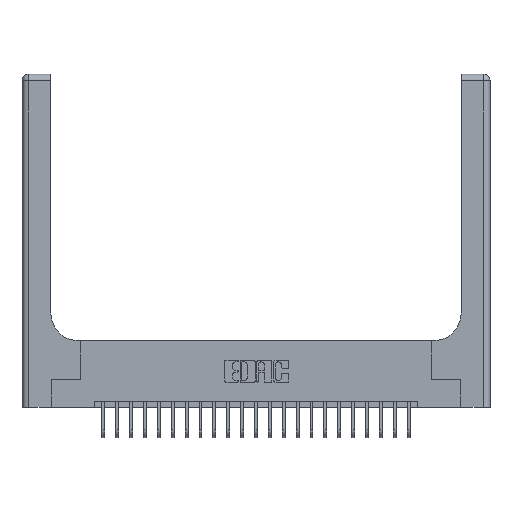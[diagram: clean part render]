
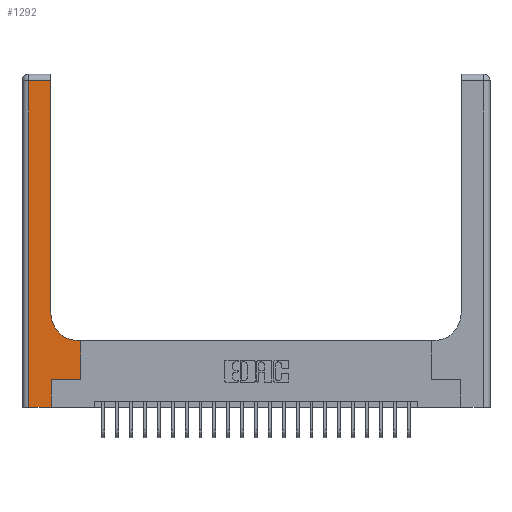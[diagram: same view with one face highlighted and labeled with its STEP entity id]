
A CAD part, top view. The second image highlights one B-rep face of the part: STEP entity #1292.
In plain terms, the highlighted planar face has unit normal (0, 0, 1).
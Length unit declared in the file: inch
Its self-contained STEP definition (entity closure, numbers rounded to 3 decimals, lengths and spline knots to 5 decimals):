
#1076 = DIRECTION ( 'NONE',  ( 0., 1., 0. ) ) ;
#1092 = EDGE_CURVE ( 'NONE', #19050, #2281, #2608, .T. ) ;
#1292 = ADVANCED_FACE ( 'NONE', ( #13601 ), #2455, .F. ) ;
#1401 = ORIENTED_EDGE ( 'NONE', *, *, #18985, .T. ) ;
#2281 = VERTEX_POINT ( 'NONE', #19230 ) ;
#2455 = PLANE ( 'NONE',  #23787 ) ;
#2608 = LINE ( 'NONE', #10828, #12054 ) ;
#2901 = VERTEX_POINT ( 'NONE', #22803 ) ;
#3121 = LINE ( 'NONE', #18926, #4268 ) ;
#3217 = ORIENTED_EDGE ( 'NONE', *, *, #4120, .T. ) ;
#3224 = ORIENTED_EDGE ( 'NONE', *, *, #18389, .T. ) ;
#3580 = ORIENTED_EDGE ( 'NONE', *, *, #6769, .T. ) ;
#3586 = CARTESIAN_POINT ( 'NONE',  ( 0.26, 0.6, 0.37 ) ) ;
#3805 = DIRECTION ( 'NONE',  ( 1., 0., 0. ) ) ;
#4120 = EDGE_CURVE ( 'NONE', #17356, #2901, #12919, .T. ) ;
#4268 = VECTOR ( 'NONE', #11097, 39.37008 ) ;
#4300 = CARTESIAN_POINT ( 'NONE',  ( 0.528, 0.6, 0.37 ) ) ;
#5118 = LINE ( 'NONE', #6899, #14669 ) ;
#5303 = VECTOR ( 'NONE', #22408, 39.37008 ) ;
#5457 = VECTOR ( 'NONE', #21172, 39.37008 ) ;
#5612 = CIRCLE ( 'NONE', #20157, 0.25 ) ;
#5939 = ORIENTED_EDGE ( 'NONE', *, *, #21942, .T. ) ;
#5987 = LINE ( 'NONE', #3586, #5457 ) ;
#6032 = VERTEX_POINT ( 'NONE', #16420 ) ;
#6052 = VERTEX_POINT ( 'NONE', #10246 ) ;
#6127 = DIRECTION ( 'NONE',  ( -1., 0., 0. ) ) ;
#6225 = ORIENTED_EDGE ( 'NONE', *, *, #16526, .T. ) ;
#6570 = EDGE_CURVE ( 'NONE', #15404, #17356, #5118, .T. ) ;
#6594 = VECTOR ( 'NONE', #12509, 39.37008 ) ;
#6769 = EDGE_CURVE ( 'NONE', #7375, #6052, #11698, .T. ) ;
#6899 = CARTESIAN_POINT ( 'NONE',  ( 0.265, 0., 0.37 ) ) ;
#7027 = CARTESIAN_POINT ( 'NONE',  ( 0.06, 2.94, 0.37 ) ) ;
#7042 = ORIENTED_EDGE ( 'NONE', *, *, #6570, .T. ) ;
#7375 = VERTEX_POINT ( 'NONE', #7027 ) ;
#7415 = VECTOR ( 'NONE', #14498, 39.37008 ) ;
#8035 = CARTESIAN_POINT ( 'NONE',  ( 0., 3., 0.37 ) ) ;
#8575 = LINE ( 'NONE', #22099, #7415 ) ;
#9048 = DIRECTION ( 'NONE',  ( 0., 1., 0. ) ) ;
#9207 = CARTESIAN_POINT ( 'NONE',  ( 0.26, 0.85, 0.37 ) ) ;
#9426 = CARTESIAN_POINT ( 'NONE',  ( 0.06, 3., 0.37 ) ) ;
#9806 = DIRECTION ( 'NONE',  ( 0., -1., 0. ) ) ;
#9816 = DIRECTION ( 'NONE',  ( 0., 0., -1. ) ) ;
#10246 = CARTESIAN_POINT ( 'NONE',  ( 0.06, 0., 0.37 ) ) ;
#10755 = EDGE_CURVE ( 'NONE', #6032, #19050, #5612, .T. ) ;
#10828 = CARTESIAN_POINT ( 'NONE',  ( 0.26, 3., 0.37 ) ) ;
#11097 = DIRECTION ( 'NONE',  ( 0., 1., 0. ) ) ;
#11698 = LINE ( 'NONE', #9426, #16715 ) ;
#12054 = VECTOR ( 'NONE', #1076, 39.37008 ) ;
#12509 = DIRECTION ( 'NONE',  ( 1., 0., 0. ) ) ;
#12919 = LINE ( 'NONE', #15192, #5303 ) ;
#13601 = FACE_OUTER_BOUND ( 'NONE', #24224, .T. ) ;
#14498 = DIRECTION ( 'NONE',  ( -1., 0., 0. ) ) ;
#14669 = VECTOR ( 'NONE', #9048, 39.37008 ) ;
#14899 = CARTESIAN_POINT ( 'NONE',  ( 0.265, 0.25, 0.37 ) ) ;
#15192 = CARTESIAN_POINT ( 'NONE',  ( 0.265, 0.25, 0.37 ) ) ;
#15404 = VERTEX_POINT ( 'NONE', #16737 ) ;
#16420 = CARTESIAN_POINT ( 'NONE',  ( 0.51, 0.6, 0.37 ) ) ;
#16526 = EDGE_CURVE ( 'NONE', #2281, #7375, #8575, .T. ) ;
#16646 = ORIENTED_EDGE ( 'NONE', *, *, #10755, .T. ) ;
#16715 = VECTOR ( 'NONE', #9806, 39.37008 ) ;
#16737 = CARTESIAN_POINT ( 'NONE',  ( 0.265, 0., 0.37 ) ) ;
#17356 = VERTEX_POINT ( 'NONE', #14899 ) ;
#18082 = CARTESIAN_POINT ( 'NONE',  ( 0., 0., 0.37 ) ) ;
#18322 = LINE ( 'NONE', #18082, #6594 ) ;
#18389 = EDGE_CURVE ( 'NONE', #21845, #6032, #5987, .T. ) ;
#18926 = CARTESIAN_POINT ( 'NONE',  ( 0.528, 0.25, 0.37 ) ) ;
#18985 = EDGE_CURVE ( 'NONE', #2901, #21845, #3121, .T. ) ;
#19050 = VERTEX_POINT ( 'NONE', #9207 ) ;
#19106 = DIRECTION ( 'NONE',  ( 0., 0., -1. ) ) ;
#19230 = CARTESIAN_POINT ( 'NONE',  ( 0.26, 2.94, 0.37 ) ) ;
#20157 = AXIS2_PLACEMENT_3D ( 'NONE', #21133, #19106, #3805 ) ;
#21133 = CARTESIAN_POINT ( 'NONE',  ( 0.51, 0.85, 0.37 ) ) ;
#21172 = DIRECTION ( 'NONE',  ( -1., 0., 0. ) ) ;
#21845 = VERTEX_POINT ( 'NONE', #4300 ) ;
#21942 = EDGE_CURVE ( 'NONE', #6052, #15404, #18322, .T. ) ;
#22099 = CARTESIAN_POINT ( 'NONE',  ( 0., 2.94, 0.37 ) ) ;
#22408 = DIRECTION ( 'NONE',  ( 1., 0., 0. ) ) ;
#22803 = CARTESIAN_POINT ( 'NONE',  ( 0.528, 0.25, 0.37 ) ) ;
#23787 = AXIS2_PLACEMENT_3D ( 'NONE', #8035, #9816, #6127 ) ;
#24224 = EDGE_LOOP ( 'NONE', ( #24398, #6225, #3580, #5939, #7042, #3217, #1401, #3224, #16646 ) ) ;
#24398 = ORIENTED_EDGE ( 'NONE', *, *, #1092, .T. ) ;
